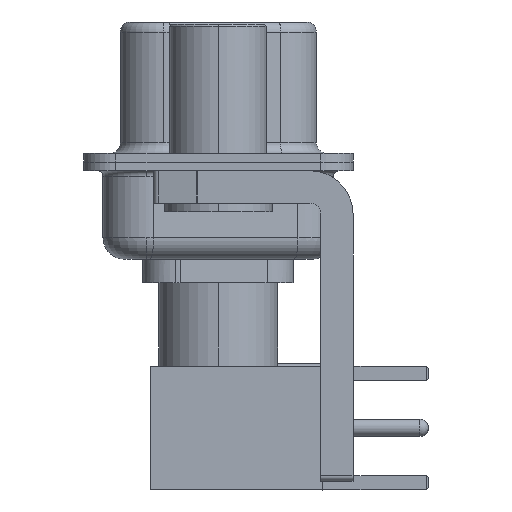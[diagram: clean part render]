
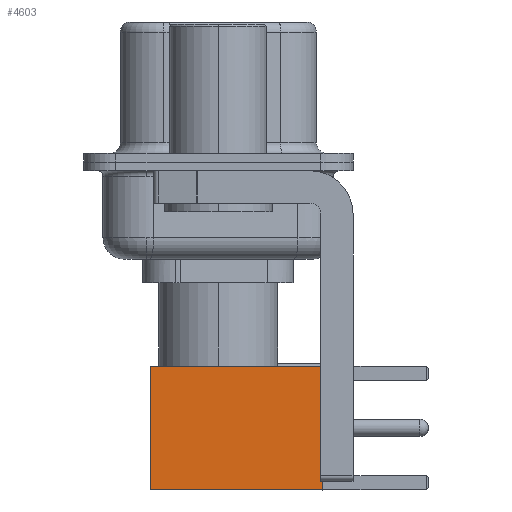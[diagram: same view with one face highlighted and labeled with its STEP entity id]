
A CAD part, left-side view. The second image highlights one B-rep face of the part: STEP entity #4603.
In plain terms, the highlighted face is planar.
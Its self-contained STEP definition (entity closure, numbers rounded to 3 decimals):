
#221 = DIRECTION ( 'NONE',  ( -1., 0., 0. ) ) ;
#891 = EDGE_CURVE ( 'NONE', #1233, #11377, #14168, .T. ) ;
#1233 = VERTEX_POINT ( 'NONE', #5134 ) ;
#1260 = DIRECTION ( 'NONE',  ( 0., 1., 0. ) ) ;
#2357 = EDGE_LOOP ( 'NONE', ( #2387, #3936, #12429, #4394 ) ) ;
#2387 = ORIENTED_EDGE ( 'NONE', *, *, #891, .T. ) ;
#2962 = EDGE_CURVE ( 'NONE', #14309, #23148, #27140, .T. ) ;
#3121 = DIRECTION ( 'NONE',  ( -1., 0., 0. ) ) ;
#3897 = DIRECTION ( 'NONE',  ( 0., 0., 1. ) ) ;
#3936 = ORIENTED_EDGE ( 'NONE', *, *, #23512, .T. ) ;
#4061 = CARTESIAN_POINT ( 'NONE',  ( 2.875, 2.875, 0. ) ) ;
#4394 = ORIENTED_EDGE ( 'NONE', *, *, #31625, .F. ) ;
#4580 = DIRECTION ( 'NONE',  ( 0., 0., -1. ) ) ;
#4603 = ADVANCED_FACE ( 'NONE', ( #16553 ), #16071, .T. ) ;
#5134 = CARTESIAN_POINT ( 'NONE',  ( 2.875, 2.875, 8. ) ) ;
#6304 = VECTOR ( 'NONE', #3121, 1000. ) ;
#7198 = AXIS2_PLACEMENT_3D ( 'NONE', #4061, #1260, #3897 ) ;
#7216 = CARTESIAN_POINT ( 'NONE',  ( -2.875, 2.875, 0. ) ) ;
#8144 = CARTESIAN_POINT ( 'NONE',  ( 2.875, 2.875, 0. ) ) ;
#10179 = CARTESIAN_POINT ( 'NONE',  ( -2.875, 2.875, 8. ) ) ;
#10509 = LINE ( 'NONE', #28481, #6304 ) ;
#10910 = CARTESIAN_POINT ( 'NONE',  ( 2.875, 2.875, 0. ) ) ;
#11377 = VERTEX_POINT ( 'NONE', #8144 ) ;
#12429 = ORIENTED_EDGE ( 'NONE', *, *, #2962, .F. ) ;
#12885 = LINE ( 'NONE', #22595, #17672 ) ;
#14168 = LINE ( 'NONE', #10910, #27090 ) ;
#14309 = VERTEX_POINT ( 'NONE', #10179 ) ;
#16071 = PLANE ( 'NONE',  #7198 ) ;
#16553 = FACE_OUTER_BOUND ( 'NONE', #2357, .T. ) ;
#17672 = VECTOR ( 'NONE', #221, 1000. ) ;
#18973 = CARTESIAN_POINT ( 'NONE',  ( -2.875, 2.875, 0. ) ) ;
#22595 = CARTESIAN_POINT ( 'NONE',  ( 0., 2.875, 0. ) ) ;
#23148 = VERTEX_POINT ( 'NONE', #18973 ) ;
#23512 = EDGE_CURVE ( 'NONE', #11377, #23148, #12885, .T. ) ;
#27090 = VECTOR ( 'NONE', #28705, 1000. ) ;
#27140 = LINE ( 'NONE', #7216, #30879 ) ;
#28481 = CARTESIAN_POINT ( 'NONE',  ( 0., 2.875, 8. ) ) ;
#28705 = DIRECTION ( 'NONE',  ( 0., 0., -1. ) ) ;
#30879 = VECTOR ( 'NONE', #4580, 1000. ) ;
#31625 = EDGE_CURVE ( 'NONE', #1233, #14309, #10509, .T. ) ;
